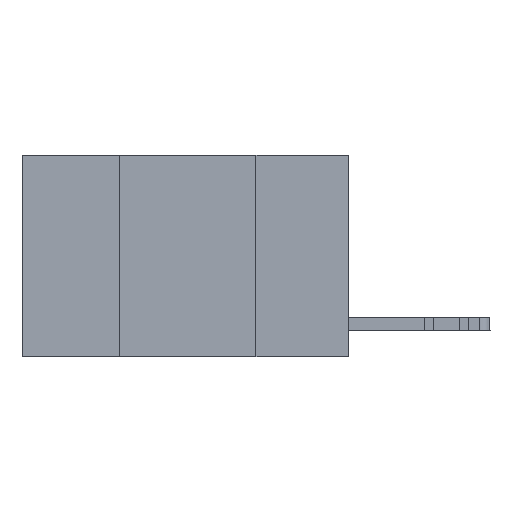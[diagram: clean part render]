
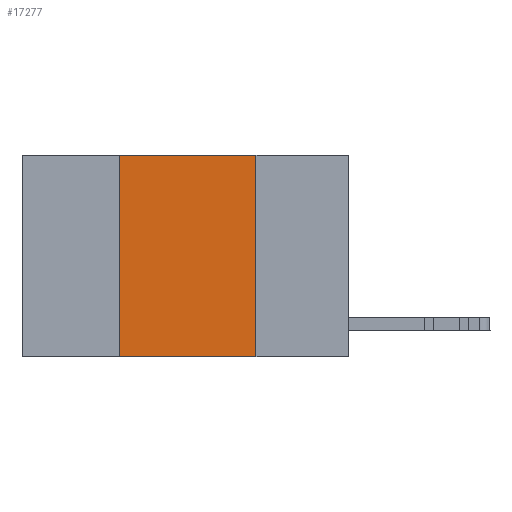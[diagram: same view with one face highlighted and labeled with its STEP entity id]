
A CAD part, left-side view. The second image highlights one B-rep face of the part: STEP entity #17277.
In plain terms, the highlighted planar face has unit normal (-1, 0, 0).
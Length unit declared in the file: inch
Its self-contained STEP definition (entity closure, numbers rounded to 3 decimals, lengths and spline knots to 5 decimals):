
#244 = LINE ( 'NONE', #20996, #24235 ) ;
#795 = VERTEX_POINT ( 'NONE', #15719 ) ;
#859 = DIRECTION ( 'NONE',  ( 0., -1., 0. ) ) ;
#2072 = VERTEX_POINT ( 'NONE', #10074 ) ;
#2536 = VECTOR ( 'NONE', #2864, 39.37008 ) ;
#2696 = LINE ( 'NONE', #3442, #23079 ) ;
#2864 = DIRECTION ( 'NONE',  ( 0., 0., 1. ) ) ;
#3442 = CARTESIAN_POINT ( 'NONE',  ( 0., 0.6, 0. ) ) ;
#5311 = VERTEX_POINT ( 'NONE', #13099 ) ;
#5516 = LINE ( 'NONE', #25968, #24054 ) ;
#7495 = LINE ( 'NONE', #16634, #2536 ) ;
#8916 = DIRECTION ( 'NONE',  ( 1., 0., 0. ) ) ;
#9030 = EDGE_CURVE ( 'NONE', #2072, #25643, #7495, .T. ) ;
#9354 = DIRECTION ( 'NONE',  ( 0., 0., -1. ) ) ;
#9359 = DIRECTION ( 'NONE',  ( 0., 0., -1. ) ) ;
#9593 = ORIENTED_EDGE ( 'NONE', *, *, #9030, .F. ) ;
#10074 = CARTESIAN_POINT ( 'NONE',  ( 0., 0.42, -0.37 ) ) ;
#11909 = EDGE_LOOP ( 'NONE', ( #17353, #18558, #9593, #24214 ) ) ;
#13099 = CARTESIAN_POINT ( 'NONE',  ( 0., 0.17, 0. ) ) ;
#13823 = CARTESIAN_POINT ( 'NONE',  ( 0., 0.6, 0. ) ) ;
#14118 = FACE_OUTER_BOUND ( 'NONE', #11909, .T. ) ;
#15719 = CARTESIAN_POINT ( 'NONE',  ( 0., 0.17, -0.37 ) ) ;
#16464 = AXIS2_PLACEMENT_3D ( 'NONE', #13823, #8916, #9359 ) ;
#16496 = EDGE_CURVE ( 'NONE', #25643, #5311, #2696, .T. ) ;
#16634 = CARTESIAN_POINT ( 'NONE',  ( 0., 0.42, 0. ) ) ;
#17021 = EDGE_CURVE ( 'NONE', #2072, #795, #5516, .T. ) ;
#17048 = DIRECTION ( 'NONE',  ( 0., -1., 0. ) ) ;
#17277 = ADVANCED_FACE ( 'NONE', ( #14118 ), #20860, .F. ) ;
#17353 = ORIENTED_EDGE ( 'NONE', *, *, #24753, .F. ) ;
#18558 = ORIENTED_EDGE ( 'NONE', *, *, #16496, .F. ) ;
#20644 = CARTESIAN_POINT ( 'NONE',  ( 0., 0.42, 0. ) ) ;
#20860 = PLANE ( 'NONE',  #16464 ) ;
#20996 = CARTESIAN_POINT ( 'NONE',  ( 0., 0.17, 0. ) ) ;
#23079 = VECTOR ( 'NONE', #17048, 39.37008 ) ;
#24054 = VECTOR ( 'NONE', #859, 39.37008 ) ;
#24214 = ORIENTED_EDGE ( 'NONE', *, *, #17021, .T. ) ;
#24235 = VECTOR ( 'NONE', #9354, 39.37008 ) ;
#24753 = EDGE_CURVE ( 'NONE', #5311, #795, #244, .T. ) ;
#25643 = VERTEX_POINT ( 'NONE', #20644 ) ;
#25968 = CARTESIAN_POINT ( 'NONE',  ( 0., 0.6, -0.37 ) ) ;
